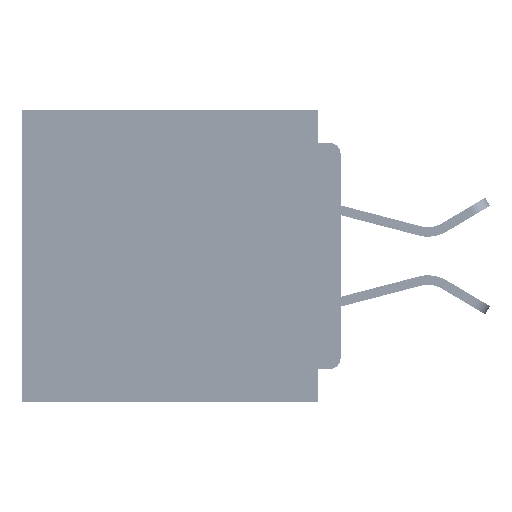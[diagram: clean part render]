
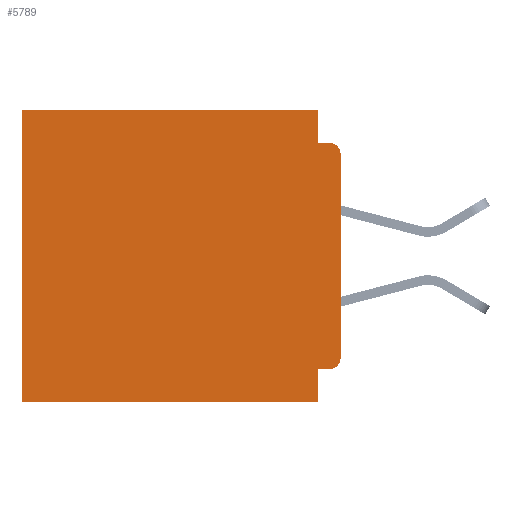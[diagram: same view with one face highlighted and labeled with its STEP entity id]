
A CAD part, left-side view. The second image highlights one B-rep face of the part: STEP entity #5789.
In plain terms, the highlighted planar face has unit normal (-1, 0, 0).
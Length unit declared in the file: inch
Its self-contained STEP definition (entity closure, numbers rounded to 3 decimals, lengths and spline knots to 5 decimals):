
#43 = CARTESIAN_POINT ( 'NONE',  ( 0.3, 0.437, -0.4 ) ) ;
#63 = EDGE_CURVE ( 'NONE', #4005, #35511, #66428, .T. ) ;
#2218 = CARTESIAN_POINT ( 'NONE',  ( 0.3, 0.015, -0.06 ) ) ;
#2681 = DIRECTION ( 'NONE',  ( 0., 1., 0. ) ) ;
#3063 = LINE ( 'NONE', #26684, #54927 ) ;
#3483 = VERTEX_POINT ( 'NONE', #38875 ) ;
#3629 = DIRECTION ( 'NONE',  ( 0., -1., 0. ) ) ;
#3792 = CARTESIAN_POINT ( 'NONE',  ( 0.3, 0., 0. ) ) ;
#4005 = VERTEX_POINT ( 'NONE', #33970 ) ;
#4084 = CARTESIAN_POINT ( 'NONE',  ( 0.3, 0.031, -0.355 ) ) ;
#5148 = VECTOR ( 'NONE', #30437, 39.37008 ) ;
#5430 = EDGE_CURVE ( 'NONE', #3483, #53891, #61943, .T. ) ;
#5465 = VECTOR ( 'NONE', #13550, 39.37008 ) ;
#5789 = ADVANCED_FACE ( 'NONE', ( #9902 ), #17743, .F. ) ;
#6007 = VERTEX_POINT ( 'NONE', #50575 ) ;
#6062 = ORIENTED_EDGE ( 'NONE', *, *, #42627, .F. ) ;
#6642 = VERTEX_POINT ( 'NONE', #43 ) ;
#6730 = CARTESIAN_POINT ( 'NONE',  ( 0.3, 0., -0.34 ) ) ;
#6974 = DIRECTION ( 'NONE',  ( 0., 0., -1. ) ) ;
#7372 = CARTESIAN_POINT ( 'NONE',  ( 0.3, 0., -0.4 ) ) ;
#7400 = DIRECTION ( 'NONE',  ( 0., 0., -1. ) ) ;
#9902 = FACE_OUTER_BOUND ( 'NONE', #56788, .T. ) ;
#10576 = VECTOR ( 'NONE', #3629, 39.37008 ) ;
#13001 = CARTESIAN_POINT ( 'NONE',  ( 0.3, 0.031, -0.045 ) ) ;
#13550 = DIRECTION ( 'NONE',  ( 0., 0., -1. ) ) ;
#13640 = DIRECTION ( 'NONE',  ( 0., 0., -1. ) ) ;
#14455 = AXIS2_PLACEMENT_3D ( 'NONE', #2218, #38371, #7400 ) ;
#15428 = VERTEX_POINT ( 'NONE', #6730 ) ;
#15917 = LINE ( 'NONE', #44573, #5465 ) ;
#15980 = VECTOR ( 'NONE', #13640, 39.37008 ) ;
#16333 = ORIENTED_EDGE ( 'NONE', *, *, #30441, .T. ) ;
#17743 = PLANE ( 'NONE',  #36445 ) ;
#18306 = EDGE_CURVE ( 'NONE', #36400, #15428, #3063, .T. ) ;
#18393 = VERTEX_POINT ( 'NONE', #32781 ) ;
#18963 = DIRECTION ( 'NONE',  ( 0., 1., 0. ) ) ;
#19384 = DIRECTION ( 'NONE',  ( -1., 0., 0. ) ) ;
#19391 = VERTEX_POINT ( 'NONE', #13001 ) ;
#20520 = VECTOR ( 'NONE', #2681, 39.37008 ) ;
#22009 = ORIENTED_EDGE ( 'NONE', *, *, #57045, .T. ) ;
#22915 = DIRECTION ( 'NONE',  ( 1., 0., 0. ) ) ;
#24305 = CIRCLE ( 'NONE', #30622, 0.015 ) ;
#24404 = ORIENTED_EDGE ( 'NONE', *, *, #25752, .F. ) ;
#25752 = EDGE_CURVE ( 'NONE', #6007, #6642, #48133, .T. ) ;
#26684 = CARTESIAN_POINT ( 'NONE',  ( 0.3, 0., -0.4 ) ) ;
#28943 = ORIENTED_EDGE ( 'NONE', *, *, #18306, .F. ) ;
#29724 = LINE ( 'NONE', #39428, #15980 ) ;
#30437 = DIRECTION ( 'NONE',  ( 0., 1., 0. ) ) ;
#30441 = EDGE_CURVE ( 'NONE', #3483, #15428, #24305, .T. ) ;
#30622 = AXIS2_PLACEMENT_3D ( 'NONE', #50452, #19384, #55716 ) ;
#32781 = CARTESIAN_POINT ( 'NONE',  ( 0.3, 0.015, -0.045 ) ) ;
#33318 = ORIENTED_EDGE ( 'NONE', *, *, #52771, .T. ) ;
#33970 = CARTESIAN_POINT ( 'NONE',  ( 0.3, 0.031, 0. ) ) ;
#34037 = VECTOR ( 'NONE', #6974, 39.37008 ) ;
#35511 = VERTEX_POINT ( 'NONE', #50178 ) ;
#35656 = CARTESIAN_POINT ( 'NONE',  ( 0.3, 0., -0.355 ) ) ;
#36400 = VERTEX_POINT ( 'NONE', #58366 ) ;
#36445 = AXIS2_PLACEMENT_3D ( 'NONE', #7372, #22915, #59308 ) ;
#38371 = DIRECTION ( 'NONE',  ( -1., 0., 0. ) ) ;
#38824 = CARTESIAN_POINT ( 'NONE',  ( 0.3, 0., -0.4 ) ) ;
#38875 = CARTESIAN_POINT ( 'NONE',  ( 0.3, 0.015, -0.355 ) ) ;
#39428 = CARTESIAN_POINT ( 'NONE',  ( 0.3, 0.031, 0. ) ) ;
#42627 = EDGE_CURVE ( 'NONE', #19391, #18393, #65764, .T. ) ;
#43384 = ORIENTED_EDGE ( 'NONE', *, *, #63, .T. ) ;
#44573 = CARTESIAN_POINT ( 'NONE',  ( 0.3, 0.031, -0.4 ) ) ;
#48133 = LINE ( 'NONE', #38824, #20520 ) ;
#48768 = ORIENTED_EDGE ( 'NONE', *, *, #62579, .F. ) ;
#50030 = CARTESIAN_POINT ( 'NONE',  ( 0.3, 0., -0.045 ) ) ;
#50178 = CARTESIAN_POINT ( 'NONE',  ( 0.3, 0.437, 0. ) ) ;
#50452 = CARTESIAN_POINT ( 'NONE',  ( 0.3, 0.015, -0.34 ) ) ;
#50575 = CARTESIAN_POINT ( 'NONE',  ( 0.3, 0.031, -0.4 ) ) ;
#52569 = VECTOR ( 'NONE', #18963, 39.37008 ) ;
#52771 = EDGE_CURVE ( 'NONE', #35511, #6642, #60124, .T. ) ;
#53891 = VERTEX_POINT ( 'NONE', #4084 ) ;
#54927 = VECTOR ( 'NONE', #63067, 39.37008 ) ;
#55716 = DIRECTION ( 'NONE',  ( 0., 0., -1. ) ) ;
#56788 = EDGE_LOOP ( 'NONE', ( #28943, #22009, #6062, #60977, #43384, #33318, #24404, #48768, #66865, #16333 ) ) ;
#57045 = EDGE_CURVE ( 'NONE', #36400, #18393, #57965, .T. ) ;
#57965 = CIRCLE ( 'NONE', #14455, 0.015 ) ;
#58366 = CARTESIAN_POINT ( 'NONE',  ( 0.3, 0., -0.06 ) ) ;
#58652 = CARTESIAN_POINT ( 'NONE',  ( 0.3, 0.437, -0.4 ) ) ;
#59308 = DIRECTION ( 'NONE',  ( 0., 0., -1. ) ) ;
#60124 = LINE ( 'NONE', #58652, #34037 ) ;
#60977 = ORIENTED_EDGE ( 'NONE', *, *, #62132, .F. ) ;
#61943 = LINE ( 'NONE', #35656, #5148 ) ;
#62132 = EDGE_CURVE ( 'NONE', #4005, #19391, #29724, .T. ) ;
#62579 = EDGE_CURVE ( 'NONE', #53891, #6007, #15917, .T. ) ;
#63067 = DIRECTION ( 'NONE',  ( 0., 0., -1. ) ) ;
#65764 = LINE ( 'NONE', #50030, #10576 ) ;
#66428 = LINE ( 'NONE', #3792, #52569 ) ;
#66865 = ORIENTED_EDGE ( 'NONE', *, *, #5430, .F. ) ;
